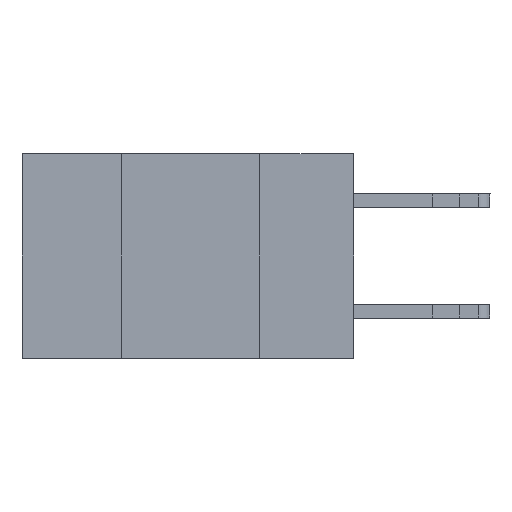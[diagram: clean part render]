
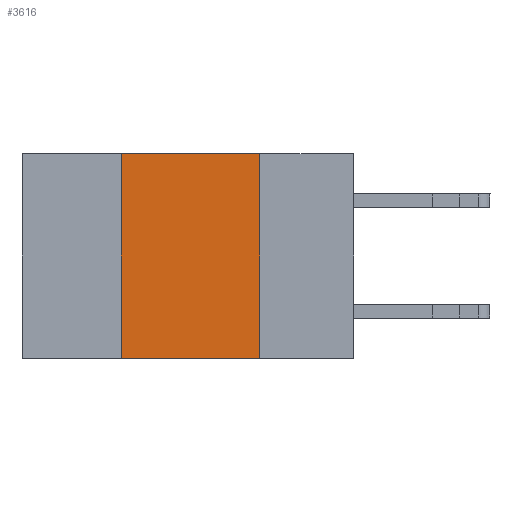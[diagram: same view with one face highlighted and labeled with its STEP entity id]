
A CAD part, left-side view. The second image highlights one B-rep face of the part: STEP entity #3616.
In plain terms, the highlighted planar face has unit normal (-1, 0, 0).
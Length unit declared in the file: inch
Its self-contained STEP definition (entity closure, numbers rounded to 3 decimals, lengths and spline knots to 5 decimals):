
#424 = AXIS2_PLACEMENT_3D ( 'NONE', #22291, #2074, #17001 ) ;
#1053 = LINE ( 'NONE', #6597, #12827 ) ;
#1637 = VECTOR ( 'NONE', #5167, 39.37008 ) ;
#2074 = DIRECTION ( 'NONE',  ( 1., 0., 0. ) ) ;
#2600 = VERTEX_POINT ( 'NONE', #15772 ) ;
#3563 = ORIENTED_EDGE ( 'NONE', *, *, #5675, .F. ) ;
#3616 = ADVANCED_FACE ( 'NONE', ( #18580 ), #13390, .F. ) ;
#3717 = CARTESIAN_POINT ( 'NONE',  ( 0., 0.42, -0.37 ) ) ;
#3781 = EDGE_CURVE ( 'NONE', #16902, #5610, #23569, .T. ) ;
#5167 = DIRECTION ( 'NONE',  ( 0., -1., 0. ) ) ;
#5610 = VERTEX_POINT ( 'NONE', #15037 ) ;
#5675 = EDGE_CURVE ( 'NONE', #16902, #2600, #1053, .T. ) ;
#6110 = DIRECTION ( 'NONE',  ( 0., -1., 0. ) ) ;
#6597 = CARTESIAN_POINT ( 'NONE',  ( 0., 0.42, 0. ) ) ;
#6779 = DIRECTION ( 'NONE',  ( 0., 0., -1. ) ) ;
#6836 = DIRECTION ( 'NONE',  ( 0., 0., 1. ) ) ;
#8495 = CARTESIAN_POINT ( 'NONE',  ( 0., 0.17, 0. ) ) ;
#8586 = VECTOR ( 'NONE', #6779, 39.37008 ) ;
#9617 = ORIENTED_EDGE ( 'NONE', *, *, #12869, .F. ) ;
#12827 = VECTOR ( 'NONE', #6836, 39.37008 ) ;
#12869 = EDGE_CURVE ( 'NONE', #13588, #5610, #17034, .T. ) ;
#13390 = PLANE ( 'NONE',  #424 ) ;
#13461 = LINE ( 'NONE', #20701, #23305 ) ;
#13588 = VERTEX_POINT ( 'NONE', #23553 ) ;
#15037 = CARTESIAN_POINT ( 'NONE',  ( 0., 0.17, -0.37 ) ) ;
#15772 = CARTESIAN_POINT ( 'NONE',  ( 0., 0.42, 0. ) ) ;
#16902 = VERTEX_POINT ( 'NONE', #3717 ) ;
#17001 = DIRECTION ( 'NONE',  ( 0., 0., -1. ) ) ;
#17034 = LINE ( 'NONE', #8495, #8586 ) ;
#17255 = ORIENTED_EDGE ( 'NONE', *, *, #22713, .F. ) ;
#18580 = FACE_OUTER_BOUND ( 'NONE', #18760, .T. ) ;
#18760 = EDGE_LOOP ( 'NONE', ( #9617, #17255, #3563, #23103 ) ) ;
#20701 = CARTESIAN_POINT ( 'NONE',  ( 0., 0.6, 0. ) ) ;
#22291 = CARTESIAN_POINT ( 'NONE',  ( 0., 0.6, 0. ) ) ;
#22713 = EDGE_CURVE ( 'NONE', #2600, #13588, #13461, .T. ) ;
#23103 = ORIENTED_EDGE ( 'NONE', *, *, #3781, .T. ) ;
#23305 = VECTOR ( 'NONE', #6110, 39.37008 ) ;
#23461 = CARTESIAN_POINT ( 'NONE',  ( 0., 0.6, -0.37 ) ) ;
#23553 = CARTESIAN_POINT ( 'NONE',  ( 0., 0.17, 0. ) ) ;
#23569 = LINE ( 'NONE', #23461, #1637 ) ;
